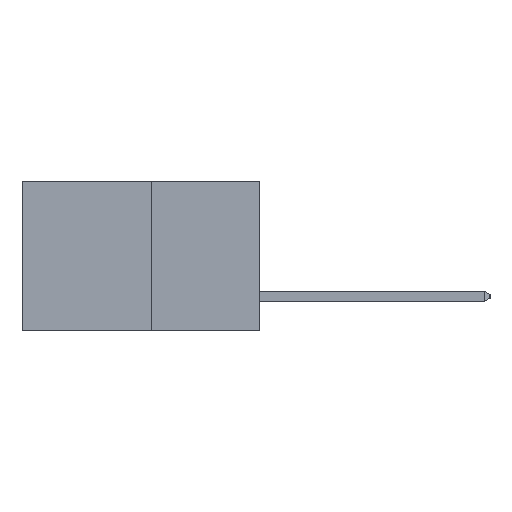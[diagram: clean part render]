
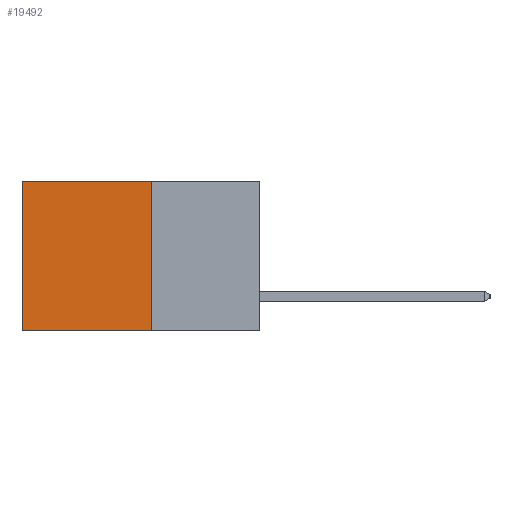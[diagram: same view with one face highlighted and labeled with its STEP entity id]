
A CAD part, left-side view. The second image highlights one B-rep face of the part: STEP entity #19492.
In plain terms, the highlighted planar face has unit normal (-1, 0, 0).
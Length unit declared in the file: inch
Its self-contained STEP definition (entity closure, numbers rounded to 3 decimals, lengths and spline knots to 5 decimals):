
#220 = LINE ( 'NONE', #13058, #8682 ) ;
#1599 = CARTESIAN_POINT ( 'NONE',  ( 0.277, 0.27, 0. ) ) ;
#1935 = ORIENTED_EDGE ( 'NONE', *, *, #5851, .T. ) ;
#2406 = VECTOR ( 'NONE', #20112, 39.37008 ) ;
#2729 = LINE ( 'NONE', #7726, #11157 ) ;
#5724 = DIRECTION ( 'NONE',  ( 0., 0., -1. ) ) ;
#5851 = EDGE_CURVE ( 'NONE', #19204, #17276, #15359, .T. ) ;
#6331 = DIRECTION ( 'NONE',  ( 0., 0., -1. ) ) ;
#7044 = AXIS2_PLACEMENT_3D ( 'NONE', #20912, #15852, #5724 ) ;
#7288 = EDGE_CURVE ( 'NONE', #19204, #12368, #220, .T. ) ;
#7726 = CARTESIAN_POINT ( 'NONE',  ( 0.277, 0.59, -0.37 ) ) ;
#8235 = CARTESIAN_POINT ( 'NONE',  ( 0.277, 0.27, 0. ) ) ;
#8591 = ORIENTED_EDGE ( 'NONE', *, *, #9205, .F. ) ;
#8682 = VECTOR ( 'NONE', #6331, 39.37008 ) ;
#8738 = FACE_OUTER_BOUND ( 'NONE', #15568, .T. ) ;
#9205 = EDGE_CURVE ( 'NONE', #12368, #14873, #13875, .T. ) ;
#11157 = VECTOR ( 'NONE', #16174, 39.37008 ) ;
#12368 = VERTEX_POINT ( 'NONE', #12682 ) ;
#12682 = CARTESIAN_POINT ( 'NONE',  ( 0.277, 0.27, -0.37 ) ) ;
#12822 = VECTOR ( 'NONE', #18124, 39.37008 ) ;
#13058 = CARTESIAN_POINT ( 'NONE',  ( 0.277, 0.27, -0.37 ) ) ;
#13875 = LINE ( 'NONE', #19822, #12822 ) ;
#14143 = PLANE ( 'NONE',  #7044 ) ;
#14513 = EDGE_CURVE ( 'NONE', #17276, #14873, #2729, .T. ) ;
#14796 = ORIENTED_EDGE ( 'NONE', *, *, #14513, .T. ) ;
#14873 = VERTEX_POINT ( 'NONE', #17118 ) ;
#15359 = LINE ( 'NONE', #8235, #2406 ) ;
#15568 = EDGE_LOOP ( 'NONE', ( #14796, #8591, #16202, #1935 ) ) ;
#15852 = DIRECTION ( 'NONE',  ( 1., 0., 0. ) ) ;
#16174 = DIRECTION ( 'NONE',  ( 0., 0., -1. ) ) ;
#16202 = ORIENTED_EDGE ( 'NONE', *, *, #7288, .F. ) ;
#17118 = CARTESIAN_POINT ( 'NONE',  ( 0.277, 0.59, -0.37 ) ) ;
#17276 = VERTEX_POINT ( 'NONE', #17500 ) ;
#17500 = CARTESIAN_POINT ( 'NONE',  ( 0.277, 0.59, 0. ) ) ;
#18124 = DIRECTION ( 'NONE',  ( 0., 1., 0. ) ) ;
#19204 = VERTEX_POINT ( 'NONE', #1599 ) ;
#19492 = ADVANCED_FACE ( 'NONE', ( #8738 ), #14143, .F. ) ;
#19822 = CARTESIAN_POINT ( 'NONE',  ( 0.277, 0.27, -0.37 ) ) ;
#20112 = DIRECTION ( 'NONE',  ( 0., 1., 0. ) ) ;
#20912 = CARTESIAN_POINT ( 'NONE',  ( 0.277, 0.27, -0.37 ) ) ;
